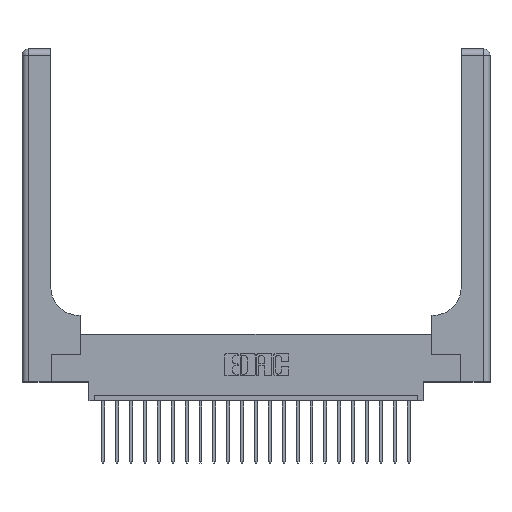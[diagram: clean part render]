
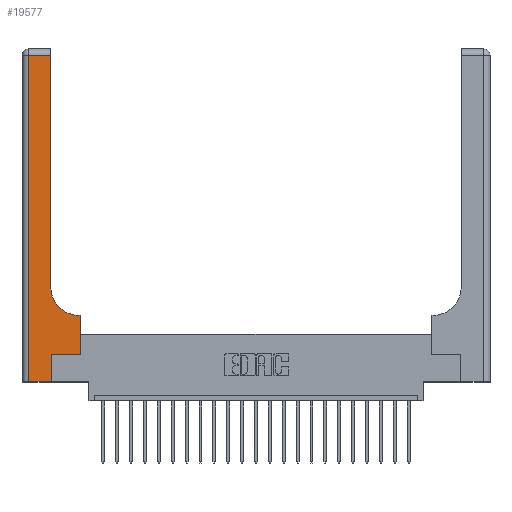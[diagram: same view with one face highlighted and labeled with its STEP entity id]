
A CAD part, top view. The second image highlights one B-rep face of the part: STEP entity #19577.
In plain terms, the highlighted planar face has unit normal (0, 0, 1).
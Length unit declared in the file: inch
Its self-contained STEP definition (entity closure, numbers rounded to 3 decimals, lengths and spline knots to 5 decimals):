
#602 = DIRECTION ( 'NONE',  ( 1., 0., 0. ) ) ;
#675 = DIRECTION ( 'NONE',  ( 0., 0., -1. ) ) ;
#937 = ORIENTED_EDGE ( 'NONE', *, *, #7155, .T. ) ;
#1546 = VERTEX_POINT ( 'NONE', #1913 ) ;
#1913 = CARTESIAN_POINT ( 'NONE',  ( 0.265, 0., 0.37 ) ) ;
#2194 = FACE_OUTER_BOUND ( 'NONE', #20887, .T. ) ;
#2465 = CARTESIAN_POINT ( 'NONE',  ( 0.528, 0.6, 0.37 ) ) ;
#2493 = DIRECTION ( 'NONE',  ( 1., 0., 0. ) ) ;
#2499 = VERTEX_POINT ( 'NONE', #8550 ) ;
#3095 = AXIS2_PLACEMENT_3D ( 'NONE', #14425, #6123, #11005 ) ;
#3914 = CARTESIAN_POINT ( 'NONE',  ( 0.528, 0.25, 0.37 ) ) ;
#4162 = EDGE_CURVE ( 'NONE', #16665, #8764, #21985, .T. ) ;
#4404 = DIRECTION ( 'NONE',  ( -1., 0., 0. ) ) ;
#5011 = LINE ( 'NONE', #20882, #8222 ) ;
#5540 = VERTEX_POINT ( 'NONE', #2465 ) ;
#5569 = EDGE_CURVE ( 'NONE', #2499, #16665, #14677, .T. ) ;
#5575 = VECTOR ( 'NONE', #19730, 39.37008 ) ;
#5592 = VECTOR ( 'NONE', #19054, 39.37008 ) ;
#5681 = CARTESIAN_POINT ( 'NONE',  ( 0.06, 0., 0.37 ) ) ;
#5724 = CARTESIAN_POINT ( 'NONE',  ( 0.51, 0.6, 0.37 ) ) ;
#6123 = DIRECTION ( 'NONE',  ( 0., 0., -1. ) ) ;
#6203 = PLANE ( 'NONE',  #3095 ) ;
#6363 = EDGE_CURVE ( 'NONE', #1546, #8418, #5011, .T. ) ;
#7006 = LINE ( 'NONE', #12290, #14750 ) ;
#7155 = EDGE_CURVE ( 'NONE', #8764, #19568, #14073, .T. ) ;
#7268 = DIRECTION ( 'NONE',  ( 0., 1., 0. ) ) ;
#8222 = VECTOR ( 'NONE', #7268, 39.37008 ) ;
#8418 = VERTEX_POINT ( 'NONE', #22143 ) ;
#8550 = CARTESIAN_POINT ( 'NONE',  ( 0.26, 0.85, 0.37 ) ) ;
#8764 = VERTEX_POINT ( 'NONE', #11498 ) ;
#9037 = VERTEX_POINT ( 'NONE', #3914 ) ;
#9575 = CARTESIAN_POINT ( 'NONE',  ( 0., 2.94, 0.37 ) ) ;
#9709 = EDGE_CURVE ( 'NONE', #18385, #2499, #10006, .T. ) ;
#10006 = CIRCLE ( 'NONE', #10881, 0.25 ) ;
#10175 = LINE ( 'NONE', #18982, #5592 ) ;
#10677 = ORIENTED_EDGE ( 'NONE', *, *, #6363, .T. ) ;
#10811 = LINE ( 'NONE', #19678, #16408 ) ;
#10881 = AXIS2_PLACEMENT_3D ( 'NONE', #21086, #675, #602 ) ;
#11005 = DIRECTION ( 'NONE',  ( -1., 0., 0. ) ) ;
#11498 = CARTESIAN_POINT ( 'NONE',  ( 0.06, 2.94, 0.37 ) ) ;
#11863 = ORIENTED_EDGE ( 'NONE', *, *, #9709, .T. ) ;
#11897 = EDGE_CURVE ( 'NONE', #5540, #18385, #19546, .T. ) ;
#12082 = ORIENTED_EDGE ( 'NONE', *, *, #20482, .T. ) ;
#12290 = CARTESIAN_POINT ( 'NONE',  ( 0.528, 0.25, 0.37 ) ) ;
#13063 = CARTESIAN_POINT ( 'NONE',  ( 0.26, 3., 0.37 ) ) ;
#13862 = DIRECTION ( 'NONE',  ( 0., 1., 0. ) ) ;
#14073 = LINE ( 'NONE', #16528, #14352 ) ;
#14352 = VECTOR ( 'NONE', #19034, 39.37008 ) ;
#14425 = CARTESIAN_POINT ( 'NONE',  ( 0., 3., 0.37 ) ) ;
#14677 = LINE ( 'NONE', #13063, #5575 ) ;
#14750 = VECTOR ( 'NONE', #13862, 39.37008 ) ;
#15722 = ORIENTED_EDGE ( 'NONE', *, *, #22080, .T. ) ;
#16104 = CARTESIAN_POINT ( 'NONE',  ( 0.26, 2.94, 0.37 ) ) ;
#16408 = VECTOR ( 'NONE', #2493, 39.37008 ) ;
#16528 = CARTESIAN_POINT ( 'NONE',  ( 0.06, 3., 0.37 ) ) ;
#16665 = VERTEX_POINT ( 'NONE', #16104 ) ;
#16975 = ORIENTED_EDGE ( 'NONE', *, *, #4162, .T. ) ;
#17927 = CARTESIAN_POINT ( 'NONE',  ( 0.26, 0.6, 0.37 ) ) ;
#18385 = VERTEX_POINT ( 'NONE', #5724 ) ;
#18452 = ORIENTED_EDGE ( 'NONE', *, *, #11897, .T. ) ;
#18911 = EDGE_CURVE ( 'NONE', #8418, #9037, #10811, .T. ) ;
#18982 = CARTESIAN_POINT ( 'NONE',  ( 0., 0., 0.37 ) ) ;
#19034 = DIRECTION ( 'NONE',  ( 0., -1., 0. ) ) ;
#19054 = DIRECTION ( 'NONE',  ( 1., 0., 0. ) ) ;
#19546 = LINE ( 'NONE', #17927, #21425 ) ;
#19568 = VERTEX_POINT ( 'NONE', #5681 ) ;
#19577 = ADVANCED_FACE ( 'NONE', ( #2194 ), #6203, .F. ) ;
#19678 = CARTESIAN_POINT ( 'NONE',  ( 0.265, 0.25, 0.37 ) ) ;
#19730 = DIRECTION ( 'NONE',  ( 0., 1., 0. ) ) ;
#19857 = DIRECTION ( 'NONE',  ( -1., 0., 0. ) ) ;
#20085 = VECTOR ( 'NONE', #19857, 39.37008 ) ;
#20482 = EDGE_CURVE ( 'NONE', #9037, #5540, #7006, .T. ) ;
#20882 = CARTESIAN_POINT ( 'NONE',  ( 0.265, 0., 0.37 ) ) ;
#20887 = EDGE_LOOP ( 'NONE', ( #22157, #16975, #937, #15722, #10677, #21581, #12082, #18452, #11863 ) ) ;
#21086 = CARTESIAN_POINT ( 'NONE',  ( 0.51, 0.85, 0.37 ) ) ;
#21425 = VECTOR ( 'NONE', #4404, 39.37008 ) ;
#21581 = ORIENTED_EDGE ( 'NONE', *, *, #18911, .T. ) ;
#21985 = LINE ( 'NONE', #9575, #20085 ) ;
#22080 = EDGE_CURVE ( 'NONE', #19568, #1546, #10175, .T. ) ;
#22143 = CARTESIAN_POINT ( 'NONE',  ( 0.265, 0.25, 0.37 ) ) ;
#22157 = ORIENTED_EDGE ( 'NONE', *, *, #5569, .T. ) ;
